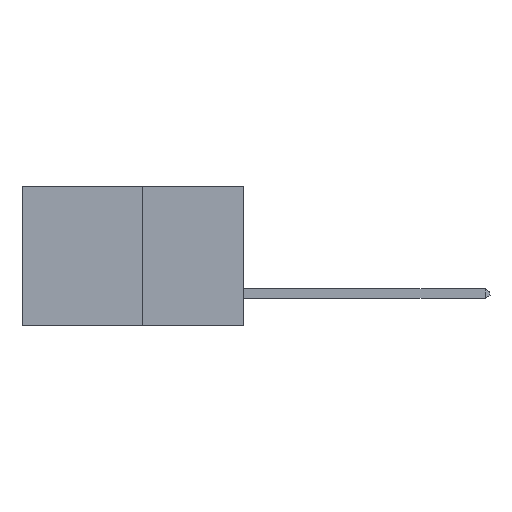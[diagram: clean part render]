
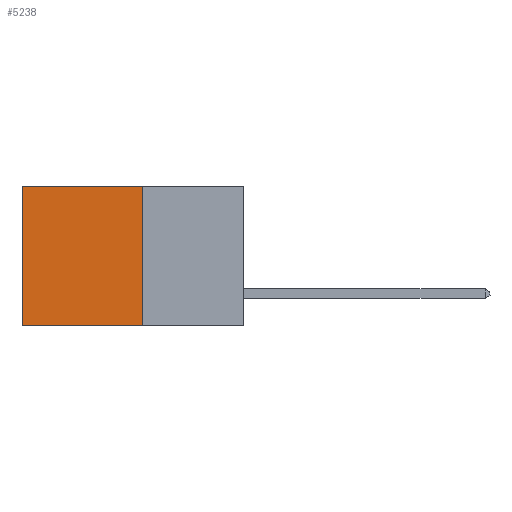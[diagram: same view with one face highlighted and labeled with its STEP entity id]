
A CAD part, left-side view. The second image highlights one B-rep face of the part: STEP entity #5238.
In plain terms, the highlighted planar face has unit normal (-1, 0, 0).
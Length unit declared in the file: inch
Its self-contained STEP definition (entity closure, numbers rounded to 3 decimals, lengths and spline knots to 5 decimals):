
#34 = CARTESIAN_POINT ( 'NONE',  ( 0.277, 0.59, -0.37 ) ) ;
#823 = DIRECTION ( 'NONE',  ( 0., 1., 0. ) ) ;
#1027 = DIRECTION ( 'NONE',  ( 0., 0., -1. ) ) ;
#1042 = CARTESIAN_POINT ( 'NONE',  ( 0.277, 0.27, 0. ) ) ;
#1413 = VECTOR ( 'NONE', #823, 39.37008 ) ;
#1440 = VECTOR ( 'NONE', #11567, 39.37008 ) ;
#1804 = AXIS2_PLACEMENT_3D ( 'NONE', #6556, #4732, #11279 ) ;
#2140 = ORIENTED_EDGE ( 'NONE', *, *, #3898, .T. ) ;
#2172 = ORIENTED_EDGE ( 'NONE', *, *, #11723, .T. ) ;
#2679 = VERTEX_POINT ( 'NONE', #8213 ) ;
#2791 = PLANE ( 'NONE',  #1804 ) ;
#2936 = ORIENTED_EDGE ( 'NONE', *, *, #8346, .F. ) ;
#2959 = ORIENTED_EDGE ( 'NONE', *, *, #3016, .F. ) ;
#3016 = EDGE_CURVE ( 'NONE', #7759, #2679, #6748, .T. ) ;
#3898 = EDGE_CURVE ( 'NONE', #10131, #4758, #3935, .T. ) ;
#3935 = LINE ( 'NONE', #1042, #1413 ) ;
#4732 = DIRECTION ( 'NONE',  ( 1., 0., 0. ) ) ;
#4758 = VERTEX_POINT ( 'NONE', #7722 ) ;
#5238 = ADVANCED_FACE ( 'NONE', ( #9477 ), #2791, .F. ) ;
#5421 = CARTESIAN_POINT ( 'NONE',  ( 0.277, 0.27, -0.37 ) ) ;
#6100 = VECTOR ( 'NONE', #11918, 39.37008 ) ;
#6556 = CARTESIAN_POINT ( 'NONE',  ( 0.277, 0.27, -0.37 ) ) ;
#6748 = LINE ( 'NONE', #11351, #1440 ) ;
#7544 = EDGE_LOOP ( 'NONE', ( #2172, #2959, #2936, #2140 ) ) ;
#7722 = CARTESIAN_POINT ( 'NONE',  ( 0.277, 0.59, 0. ) ) ;
#7759 = VERTEX_POINT ( 'NONE', #9616 ) ;
#8213 = CARTESIAN_POINT ( 'NONE',  ( 0.277, 0.59, -0.37 ) ) ;
#8346 = EDGE_CURVE ( 'NONE', #10131, #7759, #11097, .T. ) ;
#8790 = CARTESIAN_POINT ( 'NONE',  ( 0.277, 0.27, 0. ) ) ;
#9477 = FACE_OUTER_BOUND ( 'NONE', #7544, .T. ) ;
#9616 = CARTESIAN_POINT ( 'NONE',  ( 0.277, 0.27, -0.37 ) ) ;
#10131 = VERTEX_POINT ( 'NONE', #8790 ) ;
#10962 = VECTOR ( 'NONE', #1027, 39.37008 ) ;
#11097 = LINE ( 'NONE', #5421, #6100 ) ;
#11251 = LINE ( 'NONE', #34, #10962 ) ;
#11279 = DIRECTION ( 'NONE',  ( 0., 0., -1. ) ) ;
#11351 = CARTESIAN_POINT ( 'NONE',  ( 0.277, 0.27, -0.37 ) ) ;
#11567 = DIRECTION ( 'NONE',  ( 0., 1., 0. ) ) ;
#11723 = EDGE_CURVE ( 'NONE', #4758, #2679, #11251, .T. ) ;
#11918 = DIRECTION ( 'NONE',  ( 0., 0., -1. ) ) ;
